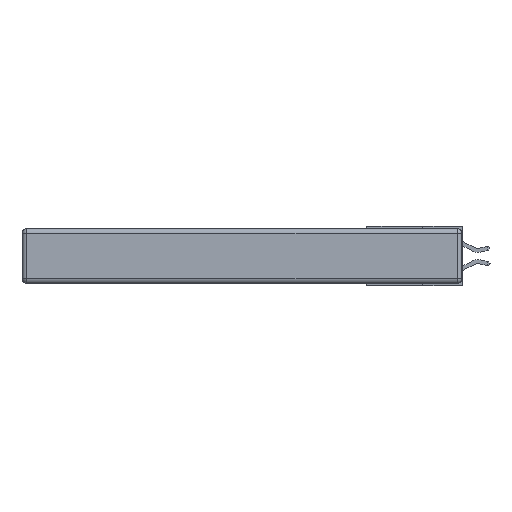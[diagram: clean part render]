
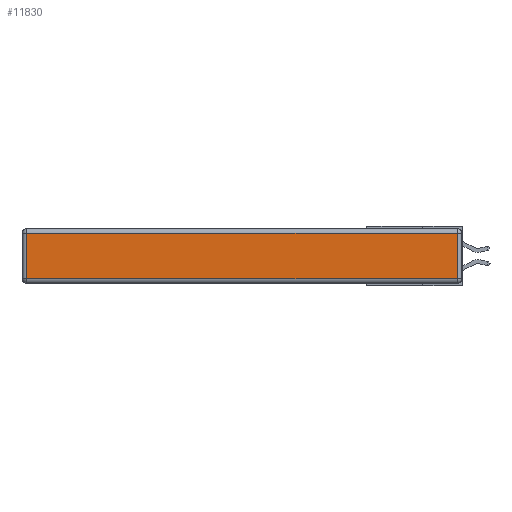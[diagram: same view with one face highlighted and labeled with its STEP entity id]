
A CAD part, left-side view. The second image highlights one B-rep face of the part: STEP entity #11830.
In plain terms, the highlighted planar face has unit normal (-1, 0, 0).
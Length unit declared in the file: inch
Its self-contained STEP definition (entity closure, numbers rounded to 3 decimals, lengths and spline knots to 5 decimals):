
#888 = DIRECTION ( 'NONE',  ( 0., -1., 0. ) ) ;
#1097 = VECTOR ( 'NONE', #888, 39.37008 ) ;
#1357 = AXIS2_PLACEMENT_3D ( 'NONE', #26690, #10483, #12517 ) ;
#1641 = LINE ( 'NONE', #28308, #4885 ) ;
#1911 = VERTEX_POINT ( 'NONE', #29888 ) ;
#2763 = ORIENTED_EDGE ( 'NONE', *, *, #4297, .T. ) ;
#2923 = DIRECTION ( 'NONE',  ( 0., 0., -1. ) ) ;
#3361 = CARTESIAN_POINT ( 'NONE',  ( 0., 0.03, -0.03 ) ) ;
#3624 = EDGE_CURVE ( 'NONE', #5887, #30359, #30145, .T. ) ;
#4006 = DIRECTION ( 'NONE',  ( 0., 0., 1. ) ) ;
#4297 = EDGE_CURVE ( 'NONE', #1911, #5887, #23869, .T. ) ;
#4885 = VECTOR ( 'NONE', #2923, 39.37008 ) ;
#5887 = VERTEX_POINT ( 'NONE', #20174 ) ;
#9143 = EDGE_LOOP ( 'NONE', ( #2763, #18986, #13098, #28458 ) ) ;
#10174 = PLANE ( 'NONE',  #1357 ) ;
#10483 = DIRECTION ( 'NONE',  ( -1., 0., 0. ) ) ;
#11830 = ADVANCED_FACE ( 'NONE', ( #25367 ), #10174, .T. ) ;
#12517 = DIRECTION ( 'NONE',  ( 0., 0., 1. ) ) ;
#13098 = ORIENTED_EDGE ( 'NONE', *, *, #19451, .T. ) ;
#16171 = CARTESIAN_POINT ( 'NONE',  ( 0., 2.72, -0.03 ) ) ;
#17606 = VECTOR ( 'NONE', #4006, 39.37008 ) ;
#18055 = CARTESIAN_POINT ( 'NONE',  ( 0., 0.03, -0.343 ) ) ;
#18986 = ORIENTED_EDGE ( 'NONE', *, *, #3624, .T. ) ;
#19451 = EDGE_CURVE ( 'NONE', #30359, #27983, #21310, .T. ) ;
#20174 = CARTESIAN_POINT ( 'NONE',  ( 0., 0.03, -0.313 ) ) ;
#21310 = LINE ( 'NONE', #21366, #24307 ) ;
#21366 = CARTESIAN_POINT ( 'NONE',  ( 0., 2.75, -0.03 ) ) ;
#22124 = CARTESIAN_POINT ( 'NONE',  ( 0., 0., -0.313 ) ) ;
#23869 = LINE ( 'NONE', #22124, #1097 ) ;
#24307 = VECTOR ( 'NONE', #28159, 39.37008 ) ;
#25367 = FACE_OUTER_BOUND ( 'NONE', #9143, .T. ) ;
#26550 = EDGE_CURVE ( 'NONE', #27983, #1911, #1641, .T. ) ;
#26690 = CARTESIAN_POINT ( 'NONE',  ( 0., 0., -0.343 ) ) ;
#27983 = VERTEX_POINT ( 'NONE', #16171 ) ;
#28159 = DIRECTION ( 'NONE',  ( 0., 1., 0. ) ) ;
#28308 = CARTESIAN_POINT ( 'NONE',  ( 0., 2.72, -0.343 ) ) ;
#28458 = ORIENTED_EDGE ( 'NONE', *, *, #26550, .T. ) ;
#29888 = CARTESIAN_POINT ( 'NONE',  ( 0., 2.72, -0.313 ) ) ;
#30145 = LINE ( 'NONE', #18055, #17606 ) ;
#30359 = VERTEX_POINT ( 'NONE', #3361 ) ;
